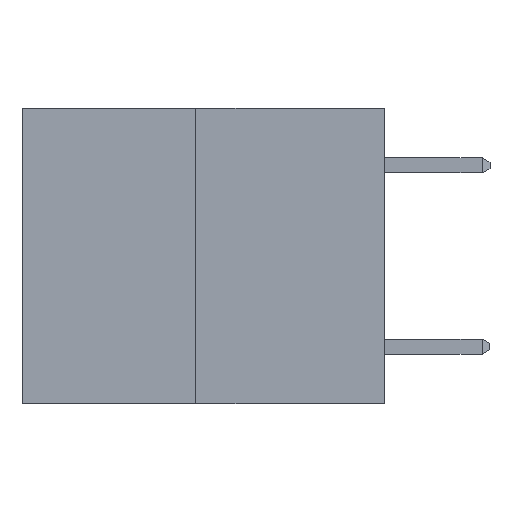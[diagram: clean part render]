
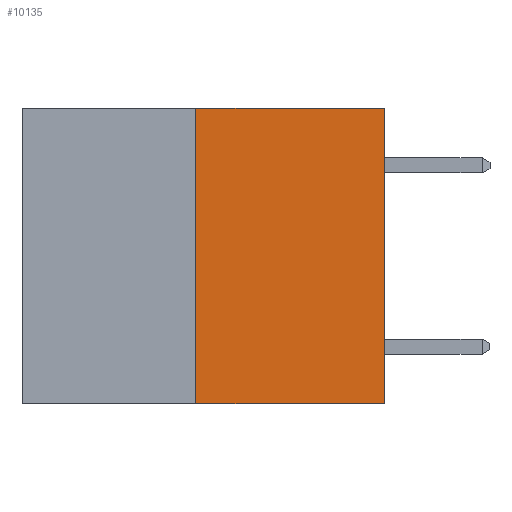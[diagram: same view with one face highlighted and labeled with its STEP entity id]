
A CAD part, left-side view. The second image highlights one B-rep face of the part: STEP entity #10135.
In plain terms, the highlighted planar face has unit normal (-1, 0, 0).
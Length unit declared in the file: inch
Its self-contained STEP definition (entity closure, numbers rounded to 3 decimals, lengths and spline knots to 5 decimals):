
#1057 = VERTEX_POINT ( 'NONE', #6097 ) ;
#1147 = VERTEX_POINT ( 'NONE', #7944 ) ;
#1592 = CARTESIAN_POINT ( 'NONE',  ( 0., 0.6, 0. ) ) ;
#2075 = CARTESIAN_POINT ( 'NONE',  ( 0., 0., 0. ) ) ;
#2130 = VECTOR ( 'NONE', #14280, 39.37008 ) ;
#2228 = ORIENTED_EDGE ( 'NONE', *, *, #11652, .F. ) ;
#2250 = ORIENTED_EDGE ( 'NONE', *, *, #4105, .T. ) ;
#2786 = VERTEX_POINT ( 'NONE', #3775 ) ;
#3617 = DIRECTION ( 'NONE',  ( 1., 0., 0. ) ) ;
#3775 = CARTESIAN_POINT ( 'NONE',  ( 0., 0., -0.49 ) ) ;
#3788 = CARTESIAN_POINT ( 'NONE',  ( 0., 0.6, 0. ) ) ;
#4105 = EDGE_CURVE ( 'NONE', #1147, #2786, #6374, .T. ) ;
#6097 = CARTESIAN_POINT ( 'NONE',  ( 0., 0.312, 0. ) ) ;
#6374 = LINE ( 'NONE', #13261, #12943 ) ;
#6447 = VERTEX_POINT ( 'NONE', #2075 ) ;
#6456 = LINE ( 'NONE', #8549, #9306 ) ;
#6500 = EDGE_LOOP ( 'NONE', ( #13581, #2250, #14980, #2228 ) ) ;
#6536 = LINE ( 'NONE', #1592, #2130 ) ;
#7463 = PLANE ( 'NONE',  #11969 ) ;
#7944 = CARTESIAN_POINT ( 'NONE',  ( 0., 0.312, -0.49 ) ) ;
#8286 = EDGE_CURVE ( 'NONE', #2786, #6447, #15974, .T. ) ;
#8549 = CARTESIAN_POINT ( 'NONE',  ( 0., 0.312, -0.49 ) ) ;
#8612 = DIRECTION ( 'NONE',  ( 0., 0., 1. ) ) ;
#9306 = VECTOR ( 'NONE', #8612, 39.37008 ) ;
#10135 = ADVANCED_FACE ( 'NONE', ( #11977 ), #7463, .F. ) ;
#11300 = DIRECTION ( 'NONE',  ( 0., 0., -1. ) ) ;
#11652 = EDGE_CURVE ( 'NONE', #1057, #6447, #6536, .T. ) ;
#11969 = AXIS2_PLACEMENT_3D ( 'NONE', #3788, #3617, #11300 ) ;
#11977 = FACE_OUTER_BOUND ( 'NONE', #6500, .T. ) ;
#12230 = VECTOR ( 'NONE', #14283, 39.37008 ) ;
#12943 = VECTOR ( 'NONE', #15795, 39.37008 ) ;
#13261 = CARTESIAN_POINT ( 'NONE',  ( 0., 0.6, -0.49 ) ) ;
#13581 = ORIENTED_EDGE ( 'NONE', *, *, #14501, .F. ) ;
#14280 = DIRECTION ( 'NONE',  ( 0., -1., 0. ) ) ;
#14283 = DIRECTION ( 'NONE',  ( 0., 0., 1. ) ) ;
#14342 = CARTESIAN_POINT ( 'NONE',  ( 0., 0., 0. ) ) ;
#14501 = EDGE_CURVE ( 'NONE', #1147, #1057, #6456, .T. ) ;
#14980 = ORIENTED_EDGE ( 'NONE', *, *, #8286, .T. ) ;
#15795 = DIRECTION ( 'NONE',  ( 0., -1., 0. ) ) ;
#15974 = LINE ( 'NONE', #14342, #12230 ) ;
